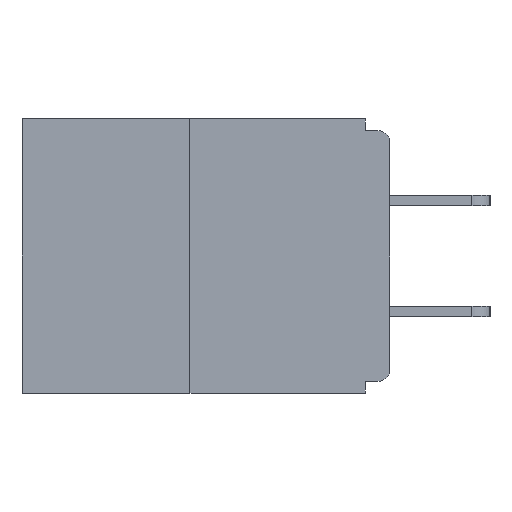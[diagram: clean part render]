
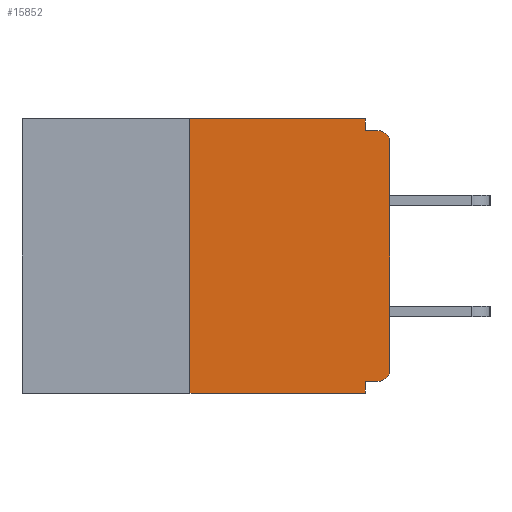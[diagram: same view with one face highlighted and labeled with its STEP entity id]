
A CAD part, left-side view. The second image highlights one B-rep face of the part: STEP entity #15852.
In plain terms, the highlighted planar face has unit normal (-1, 0, 0).
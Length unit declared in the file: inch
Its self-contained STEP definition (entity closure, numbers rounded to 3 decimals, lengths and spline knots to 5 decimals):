
#64 = LINE ( 'NONE', #7916, #699 ) ;
#182 = DIRECTION ( 'NONE',  ( 0., 0., 1. ) ) ;
#687 = CARTESIAN_POINT ( 'NONE',  ( 0., 0.015, -0.03 ) ) ;
#699 = VECTOR ( 'NONE', #182, 39.37008 ) ;
#835 = VECTOR ( 'NONE', #13825, 39.37008 ) ;
#1391 = VERTEX_POINT ( 'NONE', #20623 ) ;
#1433 = DIRECTION ( 'NONE',  ( 0., 0., -1. ) ) ;
#1527 = CARTESIAN_POINT ( 'NONE',  ( 0., 0.25, -0.343 ) ) ;
#1568 = EDGE_LOOP ( 'NONE', ( #18656, #2362, #20749, #18597, #13079, #18444, #18092, #20161, #19069, #13827 ) ) ;
#1972 = EDGE_CURVE ( 'NONE', #1391, #2606, #5741, .T. ) ;
#2362 = ORIENTED_EDGE ( 'NONE', *, *, #19003, .F. ) ;
#2606 = VERTEX_POINT ( 'NONE', #17790 ) ;
#3869 = CARTESIAN_POINT ( 'NONE',  ( 0., 0., -0.313 ) ) ;
#3963 = VECTOR ( 'NONE', #6393, 39.37008 ) ;
#4000 = DIRECTION ( 'NONE',  ( 0., 0., -1. ) ) ;
#4386 = CARTESIAN_POINT ( 'NONE',  ( 0., 0., -0.328 ) ) ;
#4648 = CARTESIAN_POINT ( 'NONE',  ( 0., 0., -0.03 ) ) ;
#4979 = VERTEX_POINT ( 'NONE', #12020 ) ;
#5221 = CIRCLE ( 'NONE', #6410, 0.015 ) ;
#5561 = DIRECTION ( 'NONE',  ( 0., 0., -1. ) ) ;
#5671 = VERTEX_POINT ( 'NONE', #3869 ) ;
#5741 = LINE ( 'NONE', #4386, #22579 ) ;
#6050 = VECTOR ( 'NONE', #5561, 39.37008 ) ;
#6287 = CARTESIAN_POINT ( 'NONE',  ( 0., 0.015, -0.015 ) ) ;
#6393 = DIRECTION ( 'NONE',  ( 0., -1., 0. ) ) ;
#6410 = AXIS2_PLACEMENT_3D ( 'NONE', #9969, #15429, #4000 ) ;
#6428 = DIRECTION ( 'NONE',  ( 0., 0., -1. ) ) ;
#6612 = CARTESIAN_POINT ( 'NONE',  ( 0., 0.031, 0. ) ) ;
#7288 = DIRECTION ( 'NONE',  ( 1., 0., 0. ) ) ;
#7428 = CARTESIAN_POINT ( 'NONE',  ( 0., 0.031, -0.343 ) ) ;
#7480 = EDGE_CURVE ( 'NONE', #4979, #18005, #12164, .T. ) ;
#7916 = CARTESIAN_POINT ( 'NONE',  ( 0., 0., 0. ) ) ;
#7992 = DIRECTION ( 'NONE',  ( 0., 1., 0. ) ) ;
#8178 = DIRECTION ( 'NONE',  ( 0., 0., -1. ) ) ;
#8306 = LINE ( 'NONE', #15894, #22530 ) ;
#8584 = VECTOR ( 'NONE', #8178, 39.37008 ) ;
#9278 = FACE_OUTER_BOUND ( 'NONE', #1568, .T. ) ;
#9417 = LINE ( 'NONE', #7428, #6050 ) ;
#9784 = VERTEX_POINT ( 'NONE', #18694 ) ;
#9797 = VERTEX_POINT ( 'NONE', #20579 ) ;
#9969 = CARTESIAN_POINT ( 'NONE',  ( 0., 0.015, -0.313 ) ) ;
#10543 = DIRECTION ( 'NONE',  ( 0., -1., 0. ) ) ;
#11793 = EDGE_CURVE ( 'NONE', #5671, #16547, #64, .T. ) ;
#12020 = CARTESIAN_POINT ( 'NONE',  ( 0., 0.031, -0.015 ) ) ;
#12123 = CARTESIAN_POINT ( 'NONE',  ( 0., 0.46, 0. ) ) ;
#12164 = LINE ( 'NONE', #19662, #21373 ) ;
#12288 = LINE ( 'NONE', #12532, #8584 ) ;
#12369 = EDGE_CURVE ( 'NONE', #9784, #22421, #23617, .T. ) ;
#12532 = CARTESIAN_POINT ( 'NONE',  ( 0., 0.031, 0. ) ) ;
#13079 = ORIENTED_EDGE ( 'NONE', *, *, #1972, .F. ) ;
#13588 = CARTESIAN_POINT ( 'NONE',  ( 0., 0.25, 0. ) ) ;
#13670 = DIRECTION ( 'NONE',  ( 0., -1., 0. ) ) ;
#13825 = DIRECTION ( 'NONE',  ( 0., 0., 1. ) ) ;
#13827 = ORIENTED_EDGE ( 'NONE', *, *, #16863, .F. ) ;
#14017 = DIRECTION ( 'NONE',  ( -1., 0., 0. ) ) ;
#15429 = DIRECTION ( 'NONE',  ( -1., 0., 0. ) ) ;
#15852 = ADVANCED_FACE ( 'NONE', ( #9278 ), #18399, .F. ) ;
#15894 = CARTESIAN_POINT ( 'NONE',  ( 0., 0.46, -0.343 ) ) ;
#16547 = VERTEX_POINT ( 'NONE', #4648 ) ;
#16863 = EDGE_CURVE ( 'NONE', #22421, #4979, #12288, .T. ) ;
#17623 = EDGE_CURVE ( 'NONE', #21907, #9797, #8306, .T. ) ;
#17790 = CARTESIAN_POINT ( 'NONE',  ( 0., 0.031, -0.328 ) ) ;
#18005 = VERTEX_POINT ( 'NONE', #6287 ) ;
#18092 = ORIENTED_EDGE ( 'NONE', *, *, #11793, .T. ) ;
#18399 = PLANE ( 'NONE',  #20941 ) ;
#18444 = ORIENTED_EDGE ( 'NONE', *, *, #19027, .T. ) ;
#18597 = ORIENTED_EDGE ( 'NONE', *, *, #20060, .F. ) ;
#18656 = ORIENTED_EDGE ( 'NONE', *, *, #12369, .F. ) ;
#18694 = CARTESIAN_POINT ( 'NONE',  ( 0., 0.25, 0. ) ) ;
#19003 = EDGE_CURVE ( 'NONE', #21907, #9784, #21070, .T. ) ;
#19027 = EDGE_CURVE ( 'NONE', #1391, #5671, #5221, .T. ) ;
#19069 = ORIENTED_EDGE ( 'NONE', *, *, #7480, .F. ) ;
#19662 = CARTESIAN_POINT ( 'NONE',  ( 0., 0., -0.015 ) ) ;
#20060 = EDGE_CURVE ( 'NONE', #2606, #9797, #9417, .T. ) ;
#20161 = ORIENTED_EDGE ( 'NONE', *, *, #23120, .T. ) ;
#20579 = CARTESIAN_POINT ( 'NONE',  ( 0., 0.031, -0.343 ) ) ;
#20623 = CARTESIAN_POINT ( 'NONE',  ( 0., 0.015, -0.328 ) ) ;
#20749 = ORIENTED_EDGE ( 'NONE', *, *, #17623, .T. ) ;
#20941 = AXIS2_PLACEMENT_3D ( 'NONE', #24386, #7288, #1433 ) ;
#21070 = LINE ( 'NONE', #13588, #835 ) ;
#21373 = VECTOR ( 'NONE', #13670, 39.37008 ) ;
#21907 = VERTEX_POINT ( 'NONE', #1527 ) ;
#22421 = VERTEX_POINT ( 'NONE', #6612 ) ;
#22530 = VECTOR ( 'NONE', #10543, 39.37008 ) ;
#22579 = VECTOR ( 'NONE', #7992, 39.37008 ) ;
#23110 = AXIS2_PLACEMENT_3D ( 'NONE', #687, #14017, #6428 ) ;
#23120 = EDGE_CURVE ( 'NONE', #16547, #18005, #23524, .T. ) ;
#23524 = CIRCLE ( 'NONE', #23110, 0.015 ) ;
#23617 = LINE ( 'NONE', #12123, #3963 ) ;
#24386 = CARTESIAN_POINT ( 'NONE',  ( 0., 0.46, 0. ) ) ;
